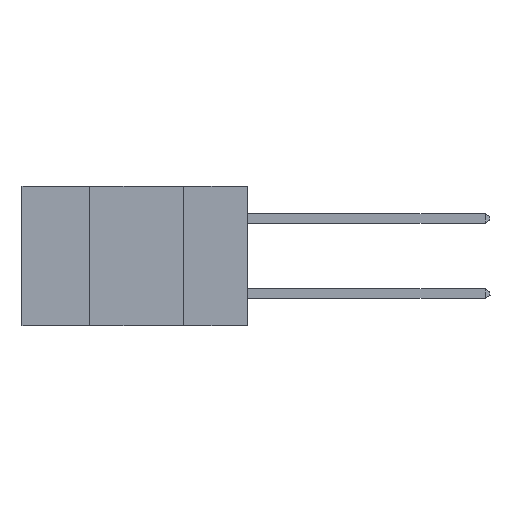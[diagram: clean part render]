
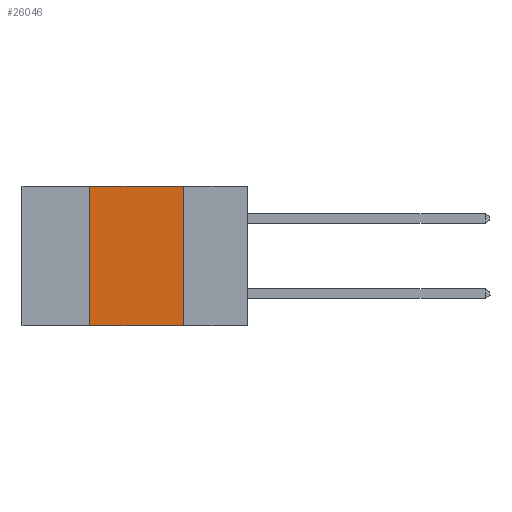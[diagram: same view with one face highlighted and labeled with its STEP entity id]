
A CAD part, left-side view. The second image highlights one B-rep face of the part: STEP entity #26046.
In plain terms, the highlighted planar face has unit normal (-1, 0, 0).
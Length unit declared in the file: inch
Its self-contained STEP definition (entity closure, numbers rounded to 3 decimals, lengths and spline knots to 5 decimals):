
#365 = EDGE_CURVE ( 'NONE', #24479, #17447, #20851, .T. ) ;
#1158 = DIRECTION ( 'NONE',  ( 0., -1., 0. ) ) ;
#2656 = DIRECTION ( 'NONE',  ( 0., -1., 0. ) ) ;
#2697 = PLANE ( 'NONE',  #8568 ) ;
#3358 = ORIENTED_EDGE ( 'NONE', *, *, #365, .T. ) ;
#4484 = DIRECTION ( 'NONE',  ( 0., 0., -1. ) ) ;
#4911 = DIRECTION ( 'NONE',  ( 1., 0., 0. ) ) ;
#7266 = CARTESIAN_POINT ( 'NONE',  ( 0., 0.42, 0. ) ) ;
#7977 = LINE ( 'NONE', #24480, #24571 ) ;
#8433 = ORIENTED_EDGE ( 'NONE', *, *, #23616, .F. ) ;
#8568 = AXIS2_PLACEMENT_3D ( 'NONE', #18114, #4911, #20243 ) ;
#8641 = VECTOR ( 'NONE', #1158, 39.37008 ) ;
#9131 = ORIENTED_EDGE ( 'NONE', *, *, #18644, .F. ) ;
#9332 = EDGE_CURVE ( 'NONE', #24479, #26174, #24151, .T. ) ;
#9539 = CARTESIAN_POINT ( 'NONE',  ( 0., 0.17, -0.37 ) ) ;
#14056 = LINE ( 'NONE', #26076, #18496 ) ;
#14765 = CARTESIAN_POINT ( 'NONE',  ( 0., 0.6, -0.37 ) ) ;
#15162 = VERTEX_POINT ( 'NONE', #24526 ) ;
#16767 = ORIENTED_EDGE ( 'NONE', *, *, #9332, .F. ) ;
#17447 = VERTEX_POINT ( 'NONE', #9539 ) ;
#17777 = FACE_OUTER_BOUND ( 'NONE', #22631, .T. ) ;
#18114 = CARTESIAN_POINT ( 'NONE',  ( 0., 0.6, 0. ) ) ;
#18496 = VECTOR ( 'NONE', #4484, 39.37008 ) ;
#18644 = EDGE_CURVE ( 'NONE', #15162, #17447, #14056, .T. ) ;
#20243 = DIRECTION ( 'NONE',  ( 0., 0., -1. ) ) ;
#20717 = CARTESIAN_POINT ( 'NONE',  ( 0., 0.42, -0.37 ) ) ;
#20851 = LINE ( 'NONE', #14765, #8641 ) ;
#22631 = EDGE_LOOP ( 'NONE', ( #9131, #8433, #16767, #3358 ) ) ;
#23487 = VECTOR ( 'NONE', #26801, 39.37008 ) ;
#23616 = EDGE_CURVE ( 'NONE', #26174, #15162, #7977, .T. ) ;
#24151 = LINE ( 'NONE', #7266, #23487 ) ;
#24479 = VERTEX_POINT ( 'NONE', #20717 ) ;
#24480 = CARTESIAN_POINT ( 'NONE',  ( 0., 0.6, 0. ) ) ;
#24526 = CARTESIAN_POINT ( 'NONE',  ( 0., 0.17, 0. ) ) ;
#24571 = VECTOR ( 'NONE', #2656, 39.37008 ) ;
#26046 = ADVANCED_FACE ( 'NONE', ( #17777 ), #2697, .F. ) ;
#26076 = CARTESIAN_POINT ( 'NONE',  ( 0., 0.17, 0. ) ) ;
#26174 = VERTEX_POINT ( 'NONE', #26949 ) ;
#26801 = DIRECTION ( 'NONE',  ( 0., 0., 1. ) ) ;
#26949 = CARTESIAN_POINT ( 'NONE',  ( 0., 0.42, 0. ) ) ;
